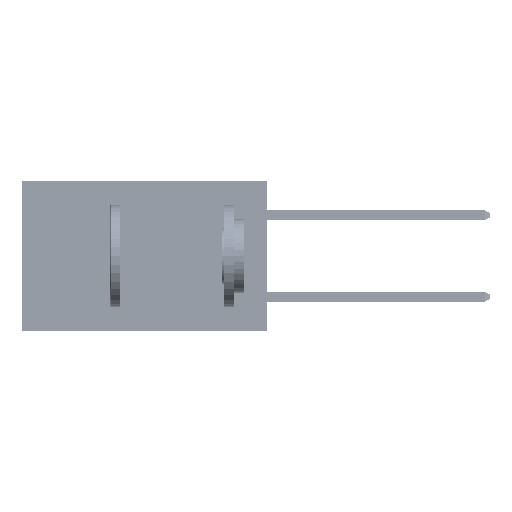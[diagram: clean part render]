
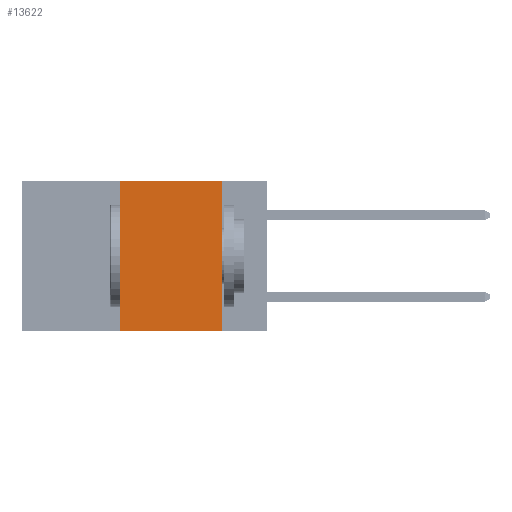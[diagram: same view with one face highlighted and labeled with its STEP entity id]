
A CAD part, left-side view. The second image highlights one B-rep face of the part: STEP entity #13622.
In plain terms, the highlighted planar face has unit normal (-1, 0, 0).
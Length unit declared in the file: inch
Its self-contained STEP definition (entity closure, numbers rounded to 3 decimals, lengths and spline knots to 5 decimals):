
#919 = CARTESIAN_POINT ( 'NONE',  ( 0., 0.36, 0. ) ) ;
#1073 = PLANE ( 'NONE',  #36667 ) ;
#1096 = LINE ( 'NONE', #48009, #3436 ) ;
#1161 = EDGE_CURVE ( 'NONE', #20148, #3993, #4642, .T. ) ;
#2940 = DIRECTION ( 'NONE',  ( 0., 0., 1. ) ) ;
#3436 = VECTOR ( 'NONE', #2940, 39.37008 ) ;
#3993 = VERTEX_POINT ( 'NONE', #7155 ) ;
#4383 = CARTESIAN_POINT ( 'NONE',  ( 0., 0.6, 0. ) ) ;
#4642 = LINE ( 'NONE', #18257, #11672 ) ;
#7155 = CARTESIAN_POINT ( 'NONE',  ( 0., 0.11, -0.37 ) ) ;
#8265 = ORIENTED_EDGE ( 'NONE', *, *, #14781, .F. ) ;
#9952 = ORIENTED_EDGE ( 'NONE', *, *, #1161, .F. ) ;
#11443 = DIRECTION ( 'NONE',  ( 0., -1., 0. ) ) ;
#11672 = VECTOR ( 'NONE', #44612, 39.37008 ) ;
#11934 = DIRECTION ( 'NONE',  ( 1., 0., 0. ) ) ;
#12008 = VECTOR ( 'NONE', #11443, 39.37008 ) ;
#13622 = ADVANCED_FACE ( 'NONE', ( #34769 ), #1073, .F. ) ;
#14191 = EDGE_LOOP ( 'NONE', ( #9952, #28365, #8265, #40324 ) ) ;
#14781 = EDGE_CURVE ( 'NONE', #32674, #29456, #1096, .T. ) ;
#18257 = CARTESIAN_POINT ( 'NONE',  ( 0., 0.11, 0. ) ) ;
#19613 = CARTESIAN_POINT ( 'NONE',  ( 0., 0.11, 0. ) ) ;
#20148 = VERTEX_POINT ( 'NONE', #19613 ) ;
#20847 = DIRECTION ( 'NONE',  ( 0., -1., 0. ) ) ;
#22152 = VECTOR ( 'NONE', #20847, 39.37008 ) ;
#28365 = ORIENTED_EDGE ( 'NONE', *, *, #30541, .F. ) ;
#29456 = VERTEX_POINT ( 'NONE', #919 ) ;
#30541 = EDGE_CURVE ( 'NONE', #29456, #20148, #46754, .T. ) ;
#32674 = VERTEX_POINT ( 'NONE', #43784 ) ;
#34769 = FACE_OUTER_BOUND ( 'NONE', #14191, .T. ) ;
#36340 = CARTESIAN_POINT ( 'NONE',  ( 0., 0.6, -0.37 ) ) ;
#36667 = AXIS2_PLACEMENT_3D ( 'NONE', #4383, #11934, #46310 ) ;
#40324 = ORIENTED_EDGE ( 'NONE', *, *, #48093, .T. ) ;
#40590 = CARTESIAN_POINT ( 'NONE',  ( 0., 0.6, 0. ) ) ;
#41620 = LINE ( 'NONE', #36340, #22152 ) ;
#43784 = CARTESIAN_POINT ( 'NONE',  ( 0., 0.36, -0.37 ) ) ;
#44612 = DIRECTION ( 'NONE',  ( 0., 0., -1. ) ) ;
#46310 = DIRECTION ( 'NONE',  ( 0., 0., -1. ) ) ;
#46754 = LINE ( 'NONE', #40590, #12008 ) ;
#48009 = CARTESIAN_POINT ( 'NONE',  ( 0., 0.36, 0. ) ) ;
#48093 = EDGE_CURVE ( 'NONE', #32674, #3993, #41620, .T. ) ;
